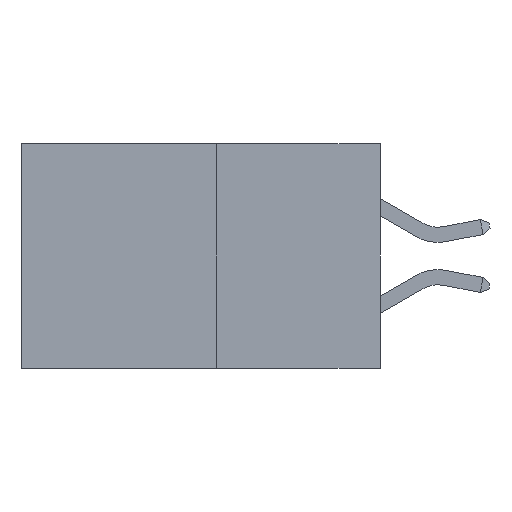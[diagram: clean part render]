
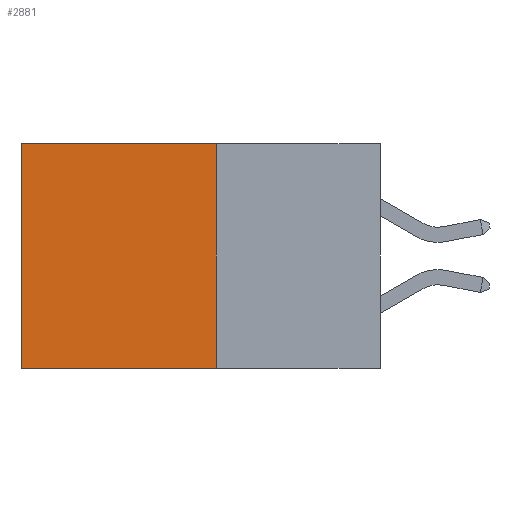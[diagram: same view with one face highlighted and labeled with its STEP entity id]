
A CAD part, left-side view. The second image highlights one B-rep face of the part: STEP entity #2881.
In plain terms, the highlighted planar face has unit normal (-1, 0, 0).
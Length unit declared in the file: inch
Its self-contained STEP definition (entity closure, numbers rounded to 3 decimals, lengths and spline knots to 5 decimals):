
#4 = LINE ( 'NONE', #335, #12024 ) ;
#335 = CARTESIAN_POINT ( 'NONE',  ( 0.277, 0.59, -0.37 ) ) ;
#1496 = DIRECTION ( 'NONE',  ( 0., 0., -1. ) ) ;
#1807 = EDGE_CURVE ( 'NONE', #9696, #5213, #9668, .T. ) ;
#2843 = LINE ( 'NONE', #11702, #3955 ) ;
#2881 = ADVANCED_FACE ( 'NONE', ( #11436 ), #4244, .F. ) ;
#3001 = CARTESIAN_POINT ( 'NONE',  ( 0.277, 0.27, -0.37 ) ) ;
#3492 = VECTOR ( 'NONE', #4889, 39.37008 ) ;
#3955 = VECTOR ( 'NONE', #11017, 39.37008 ) ;
#4190 = EDGE_CURVE ( 'NONE', #4585, #9938, #2843, .T. ) ;
#4244 = PLANE ( 'NONE',  #6056 ) ;
#4429 = VECTOR ( 'NONE', #5911, 39.37008 ) ;
#4548 = CARTESIAN_POINT ( 'NONE',  ( 0.277, 0.27, -0.37 ) ) ;
#4585 = VERTEX_POINT ( 'NONE', #12842 ) ;
#4642 = EDGE_LOOP ( 'NONE', ( #7327, #7138, #7131, #7367 ) ) ;
#4698 = CARTESIAN_POINT ( 'NONE',  ( 0.277, 0.27, -0.37 ) ) ;
#4889 = DIRECTION ( 'NONE',  ( 0., 1., 0. ) ) ;
#5005 = CARTESIAN_POINT ( 'NONE',  ( 0.277, 0.27, -0.37 ) ) ;
#5213 = VERTEX_POINT ( 'NONE', #9003 ) ;
#5911 = DIRECTION ( 'NONE',  ( 0., 0., -1. ) ) ;
#6056 = AXIS2_PLACEMENT_3D ( 'NONE', #3001, #10482, #12215 ) ;
#6130 = EDGE_CURVE ( 'NONE', #4585, #9696, #13639, .T. ) ;
#6591 = CARTESIAN_POINT ( 'NONE',  ( 0.277, 0.59, 0. ) ) ;
#6942 = EDGE_CURVE ( 'NONE', #9938, #5213, #4, .T. ) ;
#7131 = ORIENTED_EDGE ( 'NONE', *, *, #6130, .F. ) ;
#7138 = ORIENTED_EDGE ( 'NONE', *, *, #1807, .F. ) ;
#7327 = ORIENTED_EDGE ( 'NONE', *, *, #6942, .T. ) ;
#7367 = ORIENTED_EDGE ( 'NONE', *, *, #4190, .T. ) ;
#9003 = CARTESIAN_POINT ( 'NONE',  ( 0.277, 0.59, -0.37 ) ) ;
#9668 = LINE ( 'NONE', #4548, #3492 ) ;
#9696 = VERTEX_POINT ( 'NONE', #5005 ) ;
#9938 = VERTEX_POINT ( 'NONE', #6591 ) ;
#10482 = DIRECTION ( 'NONE',  ( 1., 0., 0. ) ) ;
#11017 = DIRECTION ( 'NONE',  ( 0., 1., 0. ) ) ;
#11436 = FACE_OUTER_BOUND ( 'NONE', #4642, .T. ) ;
#11702 = CARTESIAN_POINT ( 'NONE',  ( 0.277, 0.27, 0. ) ) ;
#12024 = VECTOR ( 'NONE', #1496, 39.37008 ) ;
#12215 = DIRECTION ( 'NONE',  ( 0., 0., -1. ) ) ;
#12842 = CARTESIAN_POINT ( 'NONE',  ( 0.277, 0.27, 0. ) ) ;
#13639 = LINE ( 'NONE', #4698, #4429 ) ;
